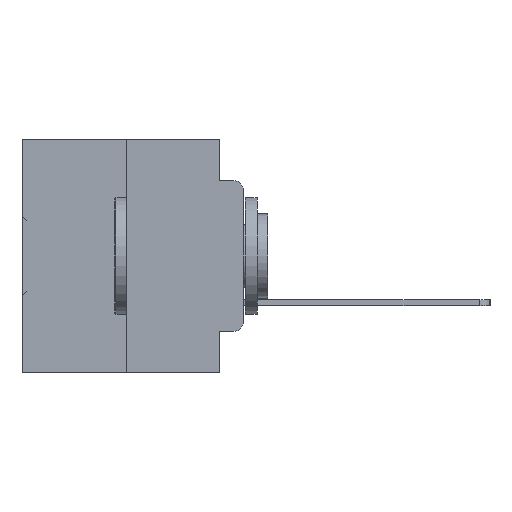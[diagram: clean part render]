
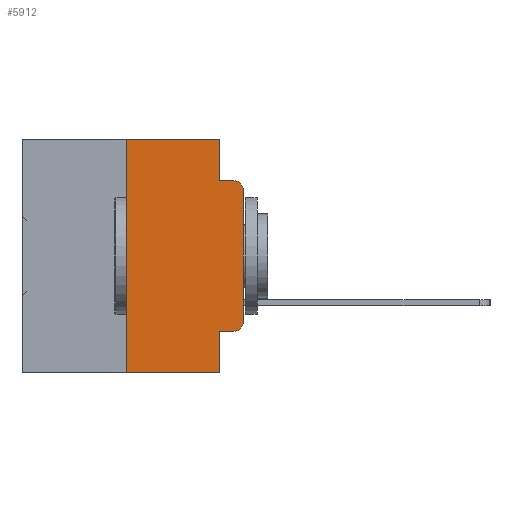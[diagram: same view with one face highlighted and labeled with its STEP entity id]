
A CAD part, left-side view. The second image highlights one B-rep face of the part: STEP entity #5912.
In plain terms, the highlighted planar face has unit normal (-1, 0, 0).
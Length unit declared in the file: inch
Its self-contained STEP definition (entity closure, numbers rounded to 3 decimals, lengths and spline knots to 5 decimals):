
#1058 = EDGE_CURVE ( 'NONE', #15559, #22243, #3815, .T. ) ;
#1097 = VECTOR ( 'NONE', #25237, 39.37008 ) ;
#1115 = EDGE_CURVE ( 'NONE', #31637, #15559, #8823, .T. ) ;
#1319 = AXIS2_PLACEMENT_3D ( 'NONE', #15125, #3512, #23876 ) ;
#1466 = CARTESIAN_POINT ( 'NONE',  ( 0., 0.02, -0.0885 ) ) ;
#2473 = DIRECTION ( 'NONE',  ( 0., -1., 0. ) ) ;
#2527 = VECTOR ( 'NONE', #22490, 39.37008 ) ;
#2541 = DIRECTION ( 'NONE',  ( 0., 0., -1. ) ) ;
#3198 = AXIS2_PLACEMENT_3D ( 'NONE', #29760, #12428, #32635 ) ;
#3216 = VECTOR ( 'NONE', #6368, 39.37008 ) ;
#3432 = CARTESIAN_POINT ( 'NONE',  ( 0., 0.473, -0.5 ) ) ;
#3512 = DIRECTION ( 'NONE',  ( 1., 0., 0. ) ) ;
#3798 = DIRECTION ( 'NONE',  ( 0., 0., -1. ) ) ;
#3815 = LINE ( 'NONE', #10328, #33745 ) ;
#3838 = ORIENTED_EDGE ( 'NONE', *, *, #33965, .T. ) ;
#4105 = LINE ( 'NONE', #14097, #18724 ) ;
#4127 = VERTEX_POINT ( 'NONE', #23869 ) ;
#5215 = ORIENTED_EDGE ( 'NONE', *, *, #8912, .F. ) ;
#5912 = ADVANCED_FACE ( 'NONE', ( #10957 ), #20999, .F. ) ;
#6173 = CARTESIAN_POINT ( 'NONE',  ( 0., 0., -0.1085 ) ) ;
#6368 = DIRECTION ( 'NONE',  ( 0., -1., 0. ) ) ;
#8823 = LINE ( 'NONE', #25203, #1097 ) ;
#8912 = EDGE_CURVE ( 'NONE', #34759, #31126, #12990, .T. ) ;
#9141 = VECTOR ( 'NONE', #24741, 39.37008 ) ;
#9321 = VECTOR ( 'NONE', #3798, 39.37008 ) ;
#9406 = CIRCLE ( 'NONE', #22050, 0.02 ) ;
#10267 = ORIENTED_EDGE ( 'NONE', *, *, #12984, .F. ) ;
#10328 = CARTESIAN_POINT ( 'NONE',  ( 0., 0.051, -0.0885 ) ) ;
#10685 = DIRECTION ( 'NONE',  ( 0., -1., 0. ) ) ;
#10709 = VERTEX_POINT ( 'NONE', #26683 ) ;
#10957 = FACE_OUTER_BOUND ( 'NONE', #36225, .T. ) ;
#11748 = EDGE_CURVE ( 'NONE', #10709, #21960, #16890, .T. ) ;
#12428 = DIRECTION ( 'NONE',  ( -1., 0., 0. ) ) ;
#12984 = EDGE_CURVE ( 'NONE', #18270, #21095, #33930, .T. ) ;
#12990 = LINE ( 'NONE', #21172, #9321 ) ;
#13781 = CARTESIAN_POINT ( 'NONE',  ( 0., 0.25, 0. ) ) ;
#14064 = EDGE_CURVE ( 'NONE', #4127, #10709, #18985, .T. ) ;
#14097 = CARTESIAN_POINT ( 'NONE',  ( 0., 0.051, -0.4115 ) ) ;
#14565 = CARTESIAN_POINT ( 'NONE',  ( 0., 0.25, -0.5 ) ) ;
#14616 = EDGE_CURVE ( 'NONE', #18270, #31126, #26418, .T. ) ;
#14815 = ORIENTED_EDGE ( 'NONE', *, *, #28363, .T. ) ;
#15125 = CARTESIAN_POINT ( 'NONE',  ( 0., 0.473, 0. ) ) ;
#15559 = VERTEX_POINT ( 'NONE', #23190 ) ;
#16454 = CARTESIAN_POINT ( 'NONE',  ( 0., 0.25, 0. ) ) ;
#16890 = LINE ( 'NONE', #18952, #9141 ) ;
#18093 = EDGE_CURVE ( 'NONE', #21095, #31637, #34276, .T. ) ;
#18270 = VERTEX_POINT ( 'NONE', #14565 ) ;
#18610 = VECTOR ( 'NONE', #36591, 39.37008 ) ;
#18724 = VECTOR ( 'NONE', #2473, 39.37008 ) ;
#18952 = CARTESIAN_POINT ( 'NONE',  ( 0., 0., 0. ) ) ;
#18985 = CIRCLE ( 'NONE', #3198, 0.02 ) ;
#19235 = CARTESIAN_POINT ( 'NONE',  ( 0., 0.051, -0.5 ) ) ;
#20019 = DIRECTION ( 'NONE',  ( -1., 0., 0. ) ) ;
#20999 = PLANE ( 'NONE',  #1319 ) ;
#21095 = VERTEX_POINT ( 'NONE', #13781 ) ;
#21172 = CARTESIAN_POINT ( 'NONE',  ( 0., 0.051, 0. ) ) ;
#21857 = CARTESIAN_POINT ( 'NONE',  ( 0., 0.473, 0. ) ) ;
#21960 = VERTEX_POINT ( 'NONE', #6173 ) ;
#22050 = AXIS2_PLACEMENT_3D ( 'NONE', #37221, #20019, #2541 ) ;
#22103 = ORIENTED_EDGE ( 'NONE', *, *, #1115, .F. ) ;
#22243 = VERTEX_POINT ( 'NONE', #1466 ) ;
#22490 = DIRECTION ( 'NONE',  ( 0., -1., 0. ) ) ;
#23190 = CARTESIAN_POINT ( 'NONE',  ( 0., 0.051, -0.0885 ) ) ;
#23869 = CARTESIAN_POINT ( 'NONE',  ( 0., 0.02, -0.4115 ) ) ;
#23876 = DIRECTION ( 'NONE',  ( 0., 0., -1. ) ) ;
#24741 = DIRECTION ( 'NONE',  ( 0., 0., 1. ) ) ;
#24775 = ORIENTED_EDGE ( 'NONE', *, *, #18093, .F. ) ;
#24993 = CARTESIAN_POINT ( 'NONE',  ( 0., 0.051, 0. ) ) ;
#25203 = CARTESIAN_POINT ( 'NONE',  ( 0., 0.051, 0. ) ) ;
#25237 = DIRECTION ( 'NONE',  ( 0., 0., -1. ) ) ;
#26418 = LINE ( 'NONE', #3432, #3216 ) ;
#26639 = CARTESIAN_POINT ( 'NONE',  ( 0., 0.051, -0.4115 ) ) ;
#26683 = CARTESIAN_POINT ( 'NONE',  ( 0., 0., -0.3915 ) ) ;
#27033 = ORIENTED_EDGE ( 'NONE', *, *, #1058, .F. ) ;
#28363 = EDGE_CURVE ( 'NONE', #34759, #4127, #4105, .T. ) ;
#29760 = CARTESIAN_POINT ( 'NONE',  ( 0., 0.02, -0.3915 ) ) ;
#30198 = ORIENTED_EDGE ( 'NONE', *, *, #14064, .T. ) ;
#31126 = VERTEX_POINT ( 'NONE', #19235 ) ;
#31637 = VERTEX_POINT ( 'NONE', #24993 ) ;
#31958 = ORIENTED_EDGE ( 'NONE', *, *, #11748, .T. ) ;
#32635 = DIRECTION ( 'NONE',  ( 0., 0., -1. ) ) ;
#33745 = VECTOR ( 'NONE', #10685, 39.37008 ) ;
#33930 = LINE ( 'NONE', #16454, #18610 ) ;
#33965 = EDGE_CURVE ( 'NONE', #21960, #22243, #9406, .T. ) ;
#34276 = LINE ( 'NONE', #21857, #2527 ) ;
#34759 = VERTEX_POINT ( 'NONE', #26639 ) ;
#35119 = ORIENTED_EDGE ( 'NONE', *, *, #14616, .T. ) ;
#36225 = EDGE_LOOP ( 'NONE', ( #31958, #3838, #27033, #22103, #24775, #10267, #35119, #5215, #14815, #30198 ) ) ;
#36591 = DIRECTION ( 'NONE',  ( 0., 0., 1. ) ) ;
#37221 = CARTESIAN_POINT ( 'NONE',  ( 0., 0.02, -0.1085 ) ) ;
